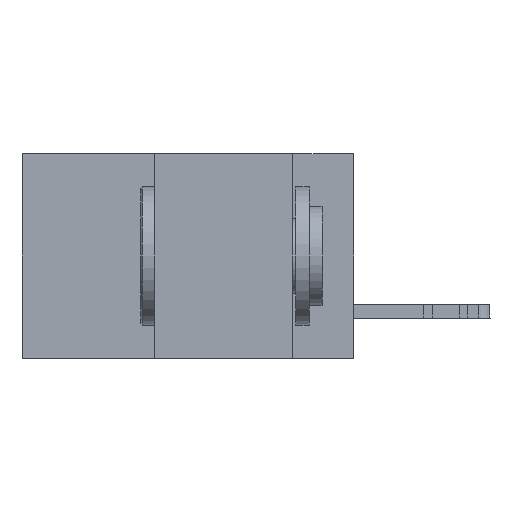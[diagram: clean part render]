
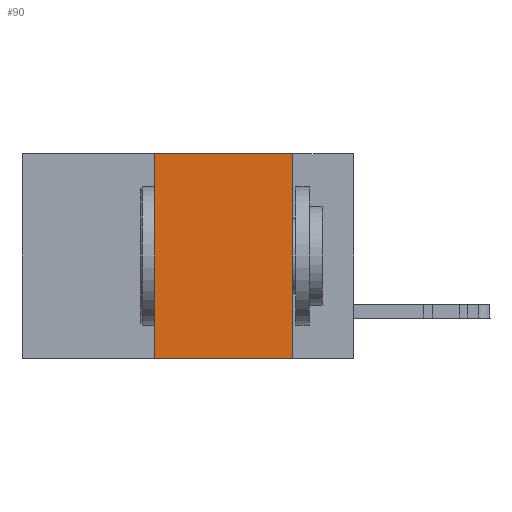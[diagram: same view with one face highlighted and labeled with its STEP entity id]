
A CAD part, left-side view. The second image highlights one B-rep face of the part: STEP entity #90.
In plain terms, the highlighted planar face has unit normal (-1, 0, 0).
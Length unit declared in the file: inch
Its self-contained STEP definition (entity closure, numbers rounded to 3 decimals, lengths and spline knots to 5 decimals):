
#90 = ADVANCED_FACE ( 'NONE', ( #32044 ), #35596, .F. ) ;
#2374 = EDGE_CURVE ( 'NONE', #14582, #34102, #34414, .T. ) ;
#3024 = DIRECTION ( 'NONE',  ( 0., -1., 0. ) ) ;
#6916 = VERTEX_POINT ( 'NONE', #16449 ) ;
#8264 = VECTOR ( 'NONE', #43204, 39.37008 ) ;
#10812 = VECTOR ( 'NONE', #3024, 39.37008 ) ;
#11996 = LINE ( 'NONE', #29141, #8264 ) ;
#13028 = CARTESIAN_POINT ( 'NONE',  ( 0., 0.11, 0. ) ) ;
#13519 = ORIENTED_EDGE ( 'NONE', *, *, #15537, .T. ) ;
#13972 = CARTESIAN_POINT ( 'NONE',  ( 0., 0.36, -0.37 ) ) ;
#14582 = VERTEX_POINT ( 'NONE', #13972 ) ;
#14970 = AXIS2_PLACEMENT_3D ( 'NONE', #21952, #31891, #39713 ) ;
#15217 = VECTOR ( 'NONE', #38459, 39.37008 ) ;
#15537 = EDGE_CURVE ( 'NONE', #14582, #6916, #19917, .T. ) ;
#15614 = ORIENTED_EDGE ( 'NONE', *, *, #2374, .F. ) ;
#16449 = CARTESIAN_POINT ( 'NONE',  ( 0., 0.11, -0.37 ) ) ;
#16599 = ORIENTED_EDGE ( 'NONE', *, *, #24976, .F. ) ;
#19173 = EDGE_CURVE ( 'NONE', #41763, #6916, #37724, .T. ) ;
#19630 = VECTOR ( 'NONE', #29815, 39.37008 ) ;
#19917 = LINE ( 'NONE', #33578, #10812 ) ;
#21952 = CARTESIAN_POINT ( 'NONE',  ( 0., 0.6, 0. ) ) ;
#24706 = CARTESIAN_POINT ( 'NONE',  ( 0., 0.36, 0. ) ) ;
#24976 = EDGE_CURVE ( 'NONE', #34102, #41763, #11996, .T. ) ;
#26724 = CARTESIAN_POINT ( 'NONE',  ( 0., 0.11, 0. ) ) ;
#27130 = CARTESIAN_POINT ( 'NONE',  ( 0., 0.36, 0. ) ) ;
#29141 = CARTESIAN_POINT ( 'NONE',  ( 0., 0.6, 0. ) ) ;
#29815 = DIRECTION ( 'NONE',  ( 0., 0., -1. ) ) ;
#31891 = DIRECTION ( 'NONE',  ( 1., 0., 0. ) ) ;
#32044 = FACE_OUTER_BOUND ( 'NONE', #34224, .T. ) ;
#33578 = CARTESIAN_POINT ( 'NONE',  ( 0., 0.6, -0.37 ) ) ;
#34102 = VERTEX_POINT ( 'NONE', #27130 ) ;
#34224 = EDGE_LOOP ( 'NONE', ( #43658, #16599, #15614, #13519 ) ) ;
#34414 = LINE ( 'NONE', #24706, #15217 ) ;
#35596 = PLANE ( 'NONE',  #14970 ) ;
#37724 = LINE ( 'NONE', #26724, #19630 ) ;
#38459 = DIRECTION ( 'NONE',  ( 0., 0., 1. ) ) ;
#39713 = DIRECTION ( 'NONE',  ( 0., 0., -1. ) ) ;
#41763 = VERTEX_POINT ( 'NONE', #13028 ) ;
#43204 = DIRECTION ( 'NONE',  ( 0., -1., 0. ) ) ;
#43658 = ORIENTED_EDGE ( 'NONE', *, *, #19173, .F. ) ;
